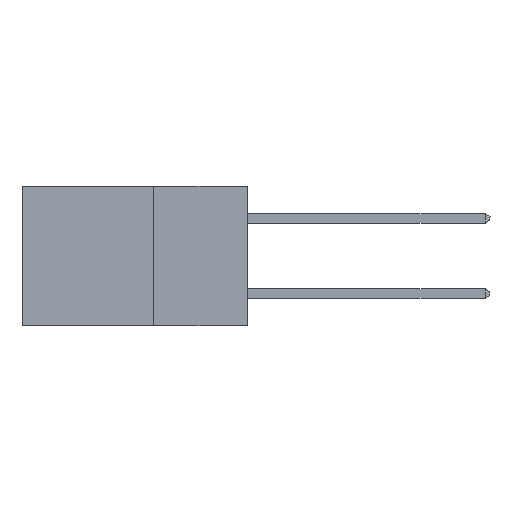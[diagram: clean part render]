
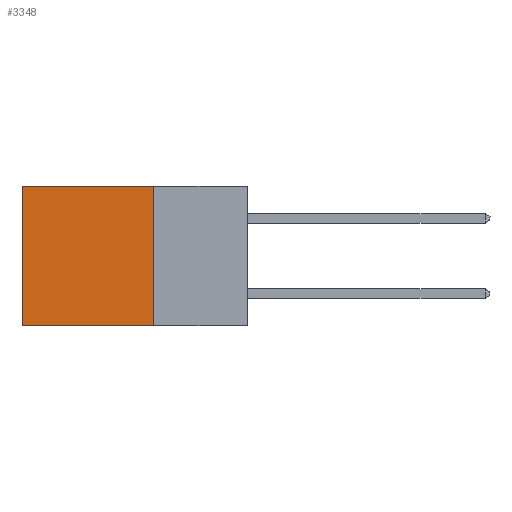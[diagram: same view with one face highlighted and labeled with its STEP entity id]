
A CAD part, left-side view. The second image highlights one B-rep face of the part: STEP entity #3348.
In plain terms, the highlighted planar face has unit normal (-1, 0, 0).
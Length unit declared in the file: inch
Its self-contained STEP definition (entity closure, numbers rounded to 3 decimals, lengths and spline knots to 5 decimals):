
#392 = ORIENTED_EDGE ( 'NONE', *, *, #4977, .T. ) ;
#393 = VECTOR ( 'NONE', #4222, 39.37008 ) ;
#548 = AXIS2_PLACEMENT_3D ( 'NONE', #9330, #2244, #4930 ) ;
#594 = DIRECTION ( 'NONE',  ( 0., 1., 0. ) ) ;
#656 = CARTESIAN_POINT ( 'NONE',  ( 0.2615, 0.25, -0.37 ) ) ;
#875 = VERTEX_POINT ( 'NONE', #2797 ) ;
#1258 = DIRECTION ( 'NONE',  ( 0., 0., -1. ) ) ;
#1452 = FACE_OUTER_BOUND ( 'NONE', #3810, .T. ) ;
#1652 = EDGE_CURVE ( 'NONE', #8712, #8370, #5752, .T. ) ;
#1800 = LINE ( 'NONE', #8770, #4048 ) ;
#2244 = DIRECTION ( 'NONE',  ( 1., 0., 0. ) ) ;
#2414 = PLANE ( 'NONE',  #548 ) ;
#2797 = CARTESIAN_POINT ( 'NONE',  ( 0.2615, 0.6, 0. ) ) ;
#3348 = ADVANCED_FACE ( 'NONE', ( #1452 ), #2414, .F. ) ;
#3508 = DIRECTION ( 'NONE',  ( 0., 1., 0. ) ) ;
#3810 = EDGE_LOOP ( 'NONE', ( #6346, #4681, #5147, #392 ) ) ;
#4048 = VECTOR ( 'NONE', #3508, 39.37008 ) ;
#4222 = DIRECTION ( 'NONE',  ( 0., 0., -1. ) ) ;
#4398 = VECTOR ( 'NONE', #594, 39.37008 ) ;
#4471 = EDGE_CURVE ( 'NONE', #8133, #8712, #10385, .T. ) ;
#4681 = ORIENTED_EDGE ( 'NONE', *, *, #1652, .F. ) ;
#4930 = DIRECTION ( 'NONE',  ( 0., 0., -1. ) ) ;
#4977 = EDGE_CURVE ( 'NONE', #8133, #875, #1800, .T. ) ;
#5147 = ORIENTED_EDGE ( 'NONE', *, *, #4471, .F. ) ;
#5225 = CARTESIAN_POINT ( 'NONE',  ( 0.2615, 0.25, -0.37 ) ) ;
#5752 = LINE ( 'NONE', #656, #4398 ) ;
#6095 = VECTOR ( 'NONE', #1258, 39.37008 ) ;
#6145 = EDGE_CURVE ( 'NONE', #875, #8370, #10841, .T. ) ;
#6346 = ORIENTED_EDGE ( 'NONE', *, *, #6145, .T. ) ;
#6731 = CARTESIAN_POINT ( 'NONE',  ( 0.2615, 0.25, 0. ) ) ;
#7372 = CARTESIAN_POINT ( 'NONE',  ( 0.2615, 0.6, -0.37 ) ) ;
#8133 = VERTEX_POINT ( 'NONE', #6731 ) ;
#8370 = VERTEX_POINT ( 'NONE', #10873 ) ;
#8712 = VERTEX_POINT ( 'NONE', #5225 ) ;
#8770 = CARTESIAN_POINT ( 'NONE',  ( 0.2615, 0.25, 0. ) ) ;
#9330 = CARTESIAN_POINT ( 'NONE',  ( 0.2615, 0.25, -0.37 ) ) ;
#9690 = CARTESIAN_POINT ( 'NONE',  ( 0.2615, 0.25, -0.37 ) ) ;
#10385 = LINE ( 'NONE', #9690, #393 ) ;
#10841 = LINE ( 'NONE', #7372, #6095 ) ;
#10873 = CARTESIAN_POINT ( 'NONE',  ( 0.2615, 0.6, -0.37 ) ) ;
